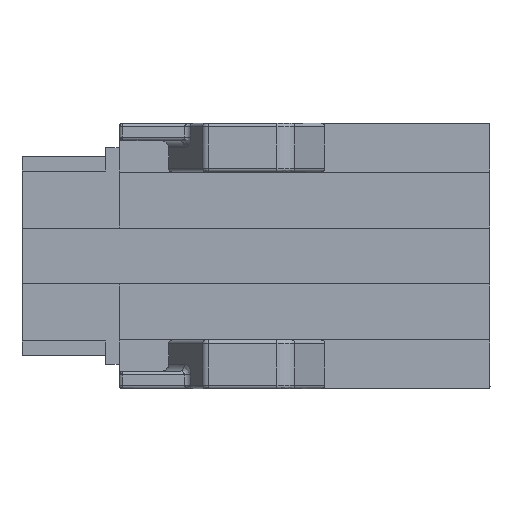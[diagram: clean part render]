
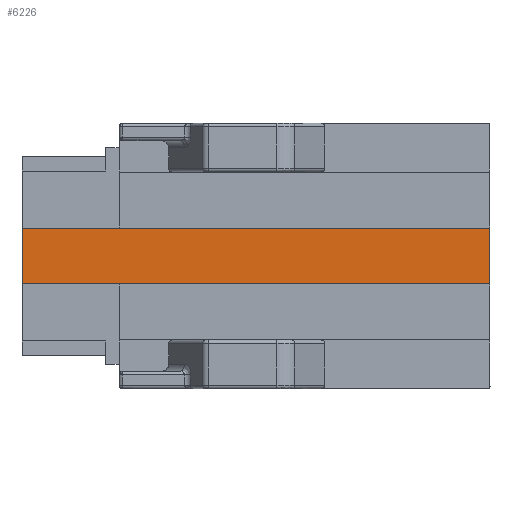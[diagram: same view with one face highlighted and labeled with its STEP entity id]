
A CAD part, left-side view. The second image highlights one B-rep face of the part: STEP entity #6226.
In plain terms, the highlighted planar face has unit normal (-1, 0, 0).
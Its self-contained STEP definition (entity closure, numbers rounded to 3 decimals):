
#1387 = VERTEX_POINT ( 'NONE', #17710 ) ;
#2583 = CARTESIAN_POINT ( 'NONE',  ( -74.875, 5.61, 5. ) ) ;
#2671 = PLANE ( 'NONE',  #3970 ) ;
#3121 = LINE ( 'NONE', #16129, #4309 ) ;
#3413 = CARTESIAN_POINT ( 'NONE',  ( -74.875, -61.29, 5. ) ) ;
#3699 = CARTESIAN_POINT ( 'NONE',  ( -74.875, -61.29, -3. ) ) ;
#3970 = AXIS2_PLACEMENT_3D ( 'NONE', #2583, #11156, #16794 ) ;
#4309 = VECTOR ( 'NONE', #6335, 1000. ) ;
#4983 = ORIENTED_EDGE ( 'NONE', *, *, #9538, .F. ) ;
#5262 = ORIENTED_EDGE ( 'NONE', *, *, #6514, .T. ) ;
#5853 = VECTOR ( 'NONE', #14402, 1000. ) ;
#6072 = EDGE_LOOP ( 'NONE', ( #6791, #17890, #4983, #5262 ) ) ;
#6226 = ADVANCED_FACE ( 'NONE', ( #6989 ), #2671, .F. ) ;
#6311 = VECTOR ( 'NONE', #8382, 1000. ) ;
#6335 = DIRECTION ( 'NONE',  ( 0., 0., 1. ) ) ;
#6514 = EDGE_CURVE ( 'NONE', #11049, #16341, #14568, .T. ) ;
#6791 = ORIENTED_EDGE ( 'NONE', *, *, #15805, .T. ) ;
#6952 = EDGE_CURVE ( 'NONE', #1387, #14099, #11343, .T. ) ;
#6989 = FACE_OUTER_BOUND ( 'NONE', #6072, .T. ) ;
#7540 = CARTESIAN_POINT ( 'NONE',  ( -74.875, 5.61, -3. ) ) ;
#8382 = DIRECTION ( 'NONE',  ( 0., -1., 0. ) ) ;
#9423 = CARTESIAN_POINT ( 'NONE',  ( -74.875, 5.61, -3. ) ) ;
#9538 = EDGE_CURVE ( 'NONE', #11049, #1387, #3121, .T. ) ;
#10519 = LINE ( 'NONE', #3413, #5853 ) ;
#11049 = VERTEX_POINT ( 'NONE', #9423 ) ;
#11156 = DIRECTION ( 'NONE',  ( 1., 0., 0. ) ) ;
#11319 = VECTOR ( 'NONE', #13185, 1000. ) ;
#11343 = LINE ( 'NONE', #16807, #6311 ) ;
#13185 = DIRECTION ( 'NONE',  ( 0., -1., 0. ) ) ;
#14099 = VERTEX_POINT ( 'NONE', #15449 ) ;
#14402 = DIRECTION ( 'NONE',  ( 0., 0., 1. ) ) ;
#14568 = LINE ( 'NONE', #7540, #11319 ) ;
#15449 = CARTESIAN_POINT ( 'NONE',  ( -74.875, -61.29, 5. ) ) ;
#15805 = EDGE_CURVE ( 'NONE', #16341, #14099, #10519, .T. ) ;
#16129 = CARTESIAN_POINT ( 'NONE',  ( -74.875, 5.61, 5. ) ) ;
#16341 = VERTEX_POINT ( 'NONE', #3699 ) ;
#16794 = DIRECTION ( 'NONE',  ( 0., 1., 0. ) ) ;
#16807 = CARTESIAN_POINT ( 'NONE',  ( -74.875, 5.61, 5. ) ) ;
#17710 = CARTESIAN_POINT ( 'NONE',  ( -74.875, 5.61, 5. ) ) ;
#17890 = ORIENTED_EDGE ( 'NONE', *, *, #6952, .F. ) ;
